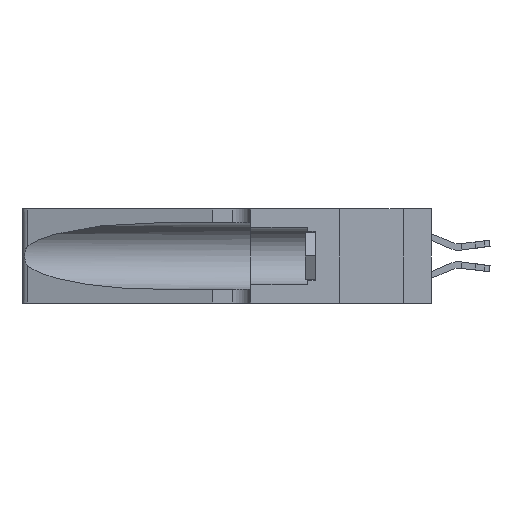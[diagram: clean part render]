
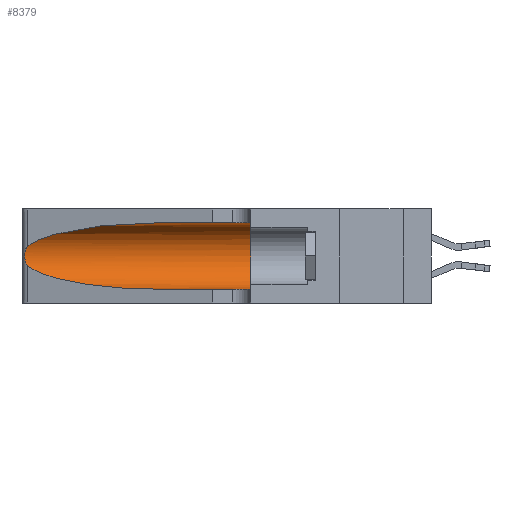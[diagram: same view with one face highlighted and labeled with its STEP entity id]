
A CAD part, left-side view. The second image highlights one B-rep face of the part: STEP entity #8379.
In plain terms, the highlighted cylindrical face has radius 3.308 mm (diameter 6.617 mm), a partial arc.
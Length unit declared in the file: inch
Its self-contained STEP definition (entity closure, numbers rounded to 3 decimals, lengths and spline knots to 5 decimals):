
#152 = FACE_OUTER_BOUND ( 'NONE', #8194, .T. ) ;
#389 = VERTEX_POINT ( 'NONE', #9393 ) ;
#1003 = CARTESIAN_POINT ( 'NONE',  ( 0.26018, 1.23835, 0.19895 ) ) ;
#1271 = CARTESIAN_POINT ( 'NONE',  ( 0.1305, 1.61858, 0.185 ) ) ;
#1298 = VERTEX_POINT ( 'NONE', #4431 ) ;
#1423 = VERTEX_POINT ( 'NONE', #6444 ) ;
#1524 = CARTESIAN_POINT ( 'NONE',  ( 0.25487, 1.22718, 0.22369 ) ) ;
#1606 = CARTESIAN_POINT ( 'NONE',  ( 0.1305, 0.35, 0.31525 ) ) ;
#1768 = CIRCLE ( 'NONE', #6850, 0.13025 ) ;
#2205 = DIRECTION ( 'NONE',  ( 0., -1., 0. ) ) ;
#2769 = DIRECTION ( 'NONE',  ( 0., -1., 0. ) ) ;
#3390 = CARTESIAN_POINT ( 'NONE',  ( 0.25487, 1.22718, 0.14631 ) ) ;
#4105 = CARTESIAN_POINT ( 'NONE',  ( 0.2373, 1.15595, 0.08982 ) ) ;
#4431 = CARTESIAN_POINT ( 'NONE',  ( 0.1305, 0.72297, 0.05475 ) ) ;
#4896 = CARTESIAN_POINT ( 'NONE',  ( 0.1305, 1.61858, 0.05475 ) ) ;
#4931 = CARTESIAN_POINT ( 'NONE',  ( 0.18966, 0.96281, 0.31525 ) ) ;
#5072 =( BOUNDED_CURVE ( )  B_SPLINE_CURVE ( 3, ( #16918, #4931, #14252, #9476 ),
 .UNSPECIFIED., .F., .T. ) 
 B_SPLINE_CURVE_WITH_KNOTS ( ( 4, 4 ),
 ( 1.5708, 2.84003 ),
 .UNSPECIFIED. ) 
 CURVE ( )  GEOMETRIC_REPRESENTATION_ITEM ( )  RATIONAL_B_SPLINE_CURVE ( ( 1., 0.87, 0.87, 1. ) ) 
 REPRESENTATION_ITEM ( '' )  );
#5703 = VERTEX_POINT ( 'NONE', #12843 ) ;
#5771 = VECTOR ( 'NONE', #8028, 39.37008 ) ;
#5982 = CARTESIAN_POINT ( 'NONE',  ( 0.1305, 0.72297, 0.05475 ) ) ;
#5998 = CARTESIAN_POINT ( 'NONE',  ( 0.25789, 1.23486, 0.15765 ) ) ;
#6444 = CARTESIAN_POINT ( 'NONE',  ( 0.1305, 0.35, 0.05475 ) ) ;
#6850 = AXIS2_PLACEMENT_3D ( 'NONE', #9496, #14070, #7668 ) ;
#7219 = CARTESIAN_POINT ( 'NONE',  ( 0.25555, 1.22993, 0.14849 ) ) ;
#7500 = EDGE_CURVE ( 'NONE', #16615, #1423, #1768, .T. ) ;
#7614 = CARTESIAN_POINT ( 'NONE',  ( 0.25555, 1.22994, 0.2215 ) ) ;
#7668 = DIRECTION ( 'NONE',  ( 0., 0., 1. ) ) ;
#7685 = CARTESIAN_POINT ( 'NONE',  ( 0.25854, 1.2359, 0.20912 ) ) ;
#8028 = DIRECTION ( 'NONE',  ( 0., -1., 0. ) ) ;
#8194 = EDGE_LOOP ( 'NONE', ( #16306, #10887, #12309, #15654, #11780, #10045 ) ) ;
#8379 = ADVANCED_FACE ( 'NONE', ( #152 ), #9619, .F. ) ;
#9393 = CARTESIAN_POINT ( 'NONE',  ( 0.1305, 0.72297, 0.31525 ) ) ;
#9476 = CARTESIAN_POINT ( 'NONE',  ( 0.25487, 1.22718, 0.22369 ) ) ;
#9496 = CARTESIAN_POINT ( 'NONE',  ( 0.1305, 0.35, 0.185 ) ) ;
#9619 = CYLINDRICAL_SURFACE ( 'NONE', #14357, 0.13025 ) ;
#9627 = EDGE_CURVE ( 'NONE', #389, #18594, #5072, .T. ) ;
#9667 = B_SPLINE_CURVE_WITH_KNOTS ( 'NONE', 3,
 ( #1524, #7614, #10800, #18030, #7685, #1003, #16879, #18470, #12335, #10675, #5998, #16805, #7219, #18402 ),
 .UNSPECIFIED., .F., .F.,
 ( 4, 2, 2, 2, 2, 2, 4 ),
 ( 0., 0.00027, 0.00053, 0.00107, 0.0016, 0.00187, 0.00214 ),
 .UNSPECIFIED. ) ;
#9761 = EDGE_CURVE ( 'NONE', #5703, #1298, #17711, .T. ) ;
#10045 = ORIENTED_EDGE ( 'NONE', *, *, #10993, .F. ) ;
#10595 = VECTOR ( 'NONE', #2205, 39.37008 ) ;
#10675 = CARTESIAN_POINT ( 'NONE',  ( 0.25856, 1.23593, 0.16098 ) ) ;
#10800 = CARTESIAN_POINT ( 'NONE',  ( 0.25639, 1.23184, 0.21858 ) ) ;
#10887 = ORIENTED_EDGE ( 'NONE', *, *, #17661, .T. ) ;
#10993 = EDGE_CURVE ( 'NONE', #389, #16615, #19748, .T. ) ;
#11780 = ORIENTED_EDGE ( 'NONE', *, *, #7500, .F. ) ;
#12070 = CARTESIAN_POINT ( 'NONE',  ( 0.18966, 0.96281, 0.05475 ) ) ;
#12309 = ORIENTED_EDGE ( 'NONE', *, *, #9761, .T. ) ;
#12335 = CARTESIAN_POINT ( 'NONE',  ( 0.26017, 1.23833, 0.17102 ) ) ;
#12355 = EDGE_CURVE ( 'NONE', #1298, #1423, #18776, .T. ) ;
#12843 = CARTESIAN_POINT ( 'NONE',  ( 0.25487, 1.22718, 0.14631 ) ) ;
#13685 = DIRECTION ( 'NONE',  ( 0., 0., -1. ) ) ;
#14070 = DIRECTION ( 'NONE',  ( 0., 1., 0. ) ) ;
#14252 = CARTESIAN_POINT ( 'NONE',  ( 0.2373, 1.15595, 0.28018 ) ) ;
#14357 = AXIS2_PLACEMENT_3D ( 'NONE', #1271, #2769, #13685 ) ;
#15654 = ORIENTED_EDGE ( 'NONE', *, *, #12355, .T. ) ;
#16306 = ORIENTED_EDGE ( 'NONE', *, *, #9627, .T. ) ;
#16374 = CARTESIAN_POINT ( 'NONE',  ( 0.25487, 1.22718, 0.22369 ) ) ;
#16615 = VERTEX_POINT ( 'NONE', #1606 ) ;
#16805 = CARTESIAN_POINT ( 'NONE',  ( 0.25639, 1.23186, 0.15144 ) ) ;
#16879 = CARTESIAN_POINT ( 'NONE',  ( 0.26075, 1.23896, 0.19203 ) ) ;
#16918 = CARTESIAN_POINT ( 'NONE',  ( 0.1305, 0.72297, 0.31525 ) ) ;
#17268 = CARTESIAN_POINT ( 'NONE',  ( 0.1305, 1.61858, 0.31525 ) ) ;
#17661 = EDGE_CURVE ( 'NONE', #18594, #5703, #9667, .T. ) ;
#17711 =( BOUNDED_CURVE ( )  B_SPLINE_CURVE ( 3, ( #3390, #4105, #12070, #5982 ),
 .UNSPECIFIED., .F., .T. ) 
 B_SPLINE_CURVE_WITH_KNOTS ( ( 4, 4 ),
 ( 3.44316, 4.71239 ),
 .UNSPECIFIED. ) 
 CURVE ( )  GEOMETRIC_REPRESENTATION_ITEM ( )  RATIONAL_B_SPLINE_CURVE ( ( 1., 0.87, 0.87, 1. ) ) 
 REPRESENTATION_ITEM ( '' )  );
#18030 = CARTESIAN_POINT ( 'NONE',  ( 0.25787, 1.23484, 0.2124 ) ) ;
#18402 = CARTESIAN_POINT ( 'NONE',  ( 0.25487, 1.22718, 0.14631 ) ) ;
#18470 = CARTESIAN_POINT ( 'NONE',  ( 0.26075, 1.23896, 0.178 ) ) ;
#18594 = VERTEX_POINT ( 'NONE', #16374 ) ;
#18776 = LINE ( 'NONE', #4896, #10595 ) ;
#19748 = LINE ( 'NONE', #17268, #5771 ) ;
